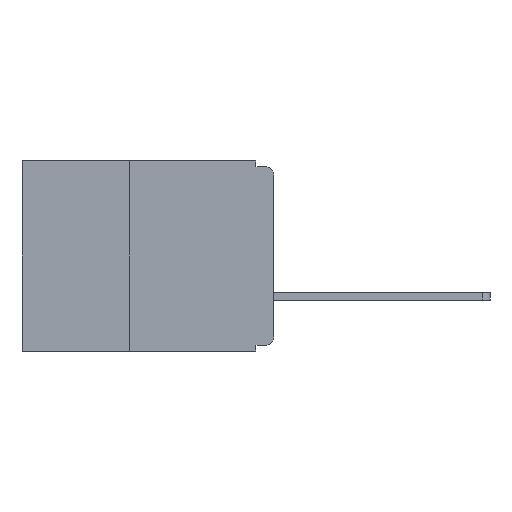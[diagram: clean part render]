
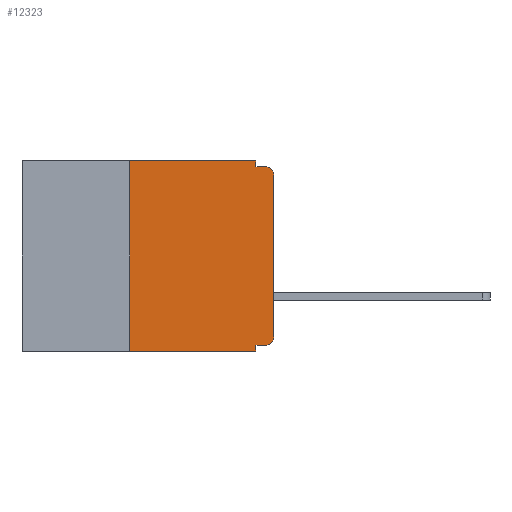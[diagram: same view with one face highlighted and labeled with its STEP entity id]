
A CAD part, left-side view. The second image highlights one B-rep face of the part: STEP entity #12323.
In plain terms, the highlighted planar face has unit normal (-1, 0, 0).
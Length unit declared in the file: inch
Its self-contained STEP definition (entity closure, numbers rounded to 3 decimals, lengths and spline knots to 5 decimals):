
#67 = CARTESIAN_POINT ( 'NONE',  ( 0., 0., 0. ) ) ;
#687 = DIRECTION ( 'NONE',  ( 0., 0., -1. ) ) ;
#1466 = ORIENTED_EDGE ( 'NONE', *, *, #14199, .T. ) ;
#1684 = AXIS2_PLACEMENT_3D ( 'NONE', #15782, #5757, #17416 ) ;
#2070 = CARTESIAN_POINT ( 'NONE',  ( 0., 0.25, -0.33 ) ) ;
#2162 = VERTEX_POINT ( 'NONE', #9610 ) ;
#2623 = EDGE_CURVE ( 'NONE', #6186, #19858, #7281, .T. ) ;
#2905 = CARTESIAN_POINT ( 'NONE',  ( 0., 0.031, -0.33 ) ) ;
#3057 = DIRECTION ( 'NONE',  ( 1., 0., 0. ) ) ;
#3375 = EDGE_CURVE ( 'NONE', #2162, #4941, #5401, .T. ) ;
#3430 = LINE ( 'NONE', #3522, #12416 ) ;
#3522 = CARTESIAN_POINT ( 'NONE',  ( 0., 0., -0.01 ) ) ;
#4018 = CARTESIAN_POINT ( 'NONE',  ( 0., 0.031, -0.01 ) ) ;
#4167 = ORIENTED_EDGE ( 'NONE', *, *, #17388, .F. ) ;
#4472 = VERTEX_POINT ( 'NONE', #8271 ) ;
#4588 = CARTESIAN_POINT ( 'NONE',  ( 0., 0.015, -0.025 ) ) ;
#4813 = CARTESIAN_POINT ( 'NONE',  ( 0., 0.015, -0.32 ) ) ;
#4941 = VERTEX_POINT ( 'NONE', #4018 ) ;
#5401 = LINE ( 'NONE', #15335, #14303 ) ;
#5554 = ORIENTED_EDGE ( 'NONE', *, *, #15615, .F. ) ;
#5757 = DIRECTION ( 'NONE',  ( -1., 0., 0. ) ) ;
#5786 = DIRECTION ( 'NONE',  ( 0., -1., 0. ) ) ;
#6186 = VERTEX_POINT ( 'NONE', #7058 ) ;
#6340 = DIRECTION ( 'NONE',  ( 0., 0., -1. ) ) ;
#6665 = VERTEX_POINT ( 'NONE', #14540 ) ;
#6700 = DIRECTION ( 'NONE',  ( 0., -1., 0. ) ) ;
#6752 = CARTESIAN_POINT ( 'NONE',  ( 0., 0., -0.32 ) ) ;
#6870 = FACE_OUTER_BOUND ( 'NONE', #10583, .T. ) ;
#7058 = CARTESIAN_POINT ( 'NONE',  ( 0., 0., -0.305 ) ) ;
#7124 = DIRECTION ( 'NONE',  ( 0., 0., 1. ) ) ;
#7281 = LINE ( 'NONE', #67, #11210 ) ;
#7400 = ORIENTED_EDGE ( 'NONE', *, *, #18376, .F. ) ;
#8271 = CARTESIAN_POINT ( 'NONE',  ( 0., 0.25, 0. ) ) ;
#8593 = VECTOR ( 'NONE', #10603, 39.37008 ) ;
#8631 = CIRCLE ( 'NONE', #1684, 0.015 ) ;
#9116 = LINE ( 'NONE', #2070, #8593 ) ;
#9209 = EDGE_CURVE ( 'NONE', #4472, #2162, #18197, .T. ) ;
#9221 = ORIENTED_EDGE ( 'NONE', *, *, #3375, .F. ) ;
#9233 = AXIS2_PLACEMENT_3D ( 'NONE', #9827, #3057, #14855 ) ;
#9402 = LINE ( 'NONE', #21124, #18211 ) ;
#9610 = CARTESIAN_POINT ( 'NONE',  ( 0., 0.031, 0. ) ) ;
#9827 = CARTESIAN_POINT ( 'NONE',  ( 0., 0.437, 0. ) ) ;
#9930 = AXIS2_PLACEMENT_3D ( 'NONE', #4588, #16343, #6340 ) ;
#10383 = VECTOR ( 'NONE', #16759, 39.37008 ) ;
#10557 = VERTEX_POINT ( 'NONE', #2905 ) ;
#10583 = EDGE_LOOP ( 'NONE', ( #16768, #19314, #4167, #9221, #15220, #7400, #12350, #17787, #5554, #1466 ) ) ;
#10586 = CARTESIAN_POINT ( 'NONE',  ( 0., 0.015, -0.01 ) ) ;
#10603 = DIRECTION ( 'NONE',  ( 0., 0., 1. ) ) ;
#10610 = CARTESIAN_POINT ( 'NONE',  ( 0., 0.031, -0.32 ) ) ;
#11191 = CARTESIAN_POINT ( 'NONE',  ( 0., 0., -0.025 ) ) ;
#11210 = VECTOR ( 'NONE', #7124, 39.37008 ) ;
#12323 = ADVANCED_FACE ( 'NONE', ( #6870 ), #13148, .F. ) ;
#12350 = ORIENTED_EDGE ( 'NONE', *, *, #12826, .T. ) ;
#12416 = VECTOR ( 'NONE', #15306, 39.37008 ) ;
#12443 = CARTESIAN_POINT ( 'NONE',  ( 0., 0.437, 0. ) ) ;
#12650 = EDGE_CURVE ( 'NONE', #19858, #14748, #18297, .T. ) ;
#12826 = EDGE_CURVE ( 'NONE', #6665, #10557, #14167, .T. ) ;
#13148 = PLANE ( 'NONE',  #9233 ) ;
#13802 = VECTOR ( 'NONE', #5786, 39.37008 ) ;
#14167 = LINE ( 'NONE', #16774, #18024 ) ;
#14199 = EDGE_CURVE ( 'NONE', #15534, #6186, #8631, .T. ) ;
#14303 = VECTOR ( 'NONE', #687, 39.37008 ) ;
#14378 = EDGE_CURVE ( 'NONE', #16381, #10557, #9402, .T. ) ;
#14540 = CARTESIAN_POINT ( 'NONE',  ( 0., 0.25, -0.33 ) ) ;
#14598 = DIRECTION ( 'NONE',  ( 0., 0., -1. ) ) ;
#14748 = VERTEX_POINT ( 'NONE', #10586 ) ;
#14855 = DIRECTION ( 'NONE',  ( 0., 0., -1. ) ) ;
#15220 = ORIENTED_EDGE ( 'NONE', *, *, #9209, .F. ) ;
#15306 = DIRECTION ( 'NONE',  ( 0., -1., 0. ) ) ;
#15335 = CARTESIAN_POINT ( 'NONE',  ( 0., 0.031, 0. ) ) ;
#15534 = VERTEX_POINT ( 'NONE', #4813 ) ;
#15615 = EDGE_CURVE ( 'NONE', #15534, #16381, #19187, .T. ) ;
#15782 = CARTESIAN_POINT ( 'NONE',  ( 0., 0.015, -0.305 ) ) ;
#16343 = DIRECTION ( 'NONE',  ( -1., 0., 0. ) ) ;
#16381 = VERTEX_POINT ( 'NONE', #10610 ) ;
#16759 = DIRECTION ( 'NONE',  ( 0., 1., 0. ) ) ;
#16768 = ORIENTED_EDGE ( 'NONE', *, *, #2623, .T. ) ;
#16774 = CARTESIAN_POINT ( 'NONE',  ( 0., 0.437, -0.33 ) ) ;
#17388 = EDGE_CURVE ( 'NONE', #4941, #14748, #3430, .T. ) ;
#17416 = DIRECTION ( 'NONE',  ( 0., 0., -1. ) ) ;
#17787 = ORIENTED_EDGE ( 'NONE', *, *, #14378, .F. ) ;
#18024 = VECTOR ( 'NONE', #6700, 39.37008 ) ;
#18197 = LINE ( 'NONE', #12443, #13802 ) ;
#18211 = VECTOR ( 'NONE', #14598, 39.37008 ) ;
#18297 = CIRCLE ( 'NONE', #9930, 0.015 ) ;
#18376 = EDGE_CURVE ( 'NONE', #6665, #4472, #9116, .T. ) ;
#19187 = LINE ( 'NONE', #6752, #10383 ) ;
#19314 = ORIENTED_EDGE ( 'NONE', *, *, #12650, .T. ) ;
#19858 = VERTEX_POINT ( 'NONE', #11191 ) ;
#21124 = CARTESIAN_POINT ( 'NONE',  ( 0., 0.031, -0.33 ) ) ;
